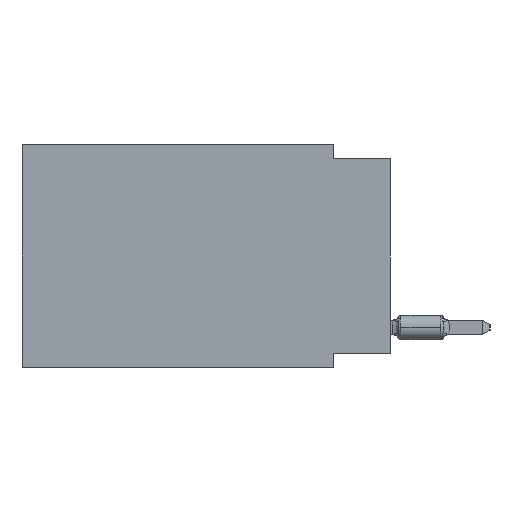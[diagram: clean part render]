
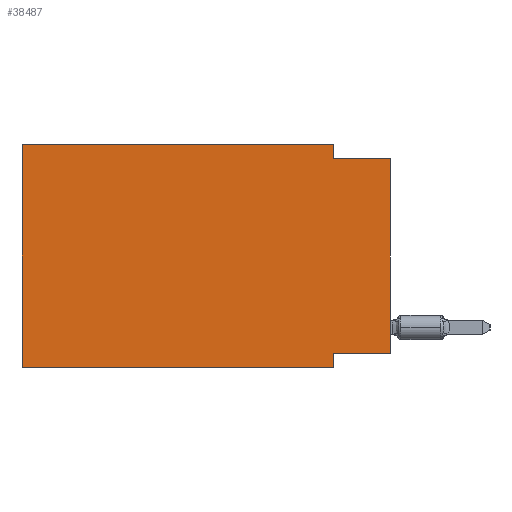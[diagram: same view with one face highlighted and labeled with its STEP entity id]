
A CAD part, left-side view. The second image highlights one B-rep face of the part: STEP entity #38487.
In plain terms, the highlighted planar face has unit normal (-1, 0, 0).
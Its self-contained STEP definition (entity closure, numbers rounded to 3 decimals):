
#952 = ORIENTED_EDGE ( 'NONE', *, *, #37551, .T. ) ;
#1107 = EDGE_CURVE ( 'NONE', #49571, #33872, #34606, .T. ) ;
#1662 = CARTESIAN_POINT ( 'NONE',  ( 0., 0., -0.635 ) ) ;
#1802 = CARTESIAN_POINT ( 'NONE',  ( 0., 16.383, -9.906 ) ) ;
#3372 = CARTESIAN_POINT ( 'NONE',  ( 0., 16.383, -9.906 ) ) ;
#3606 = CARTESIAN_POINT ( 'NONE',  ( 0., 16.383, 0. ) ) ;
#4074 = CARTESIAN_POINT ( 'NONE',  ( 0., 2.54, -9.906 ) ) ;
#4396 = CARTESIAN_POINT ( 'NONE',  ( 0., 16.383, 0. ) ) ;
#4826 = DIRECTION ( 'NONE',  ( 0., 0., -1. ) ) ;
#4965 = ORIENTED_EDGE ( 'NONE', *, *, #41860, .F. ) ;
#5560 = VECTOR ( 'NONE', #36702, 1000. ) ;
#5697 = VECTOR ( 'NONE', #9865, 1000. ) ;
#5885 = LINE ( 'NONE', #4396, #5697 ) ;
#6963 = VERTEX_POINT ( 'NONE', #3372 ) ;
#7174 = PLANE ( 'NONE',  #14794 ) ;
#7395 = ORIENTED_EDGE ( 'NONE', *, *, #29370, .F. ) ;
#7616 = ORIENTED_EDGE ( 'NONE', *, *, #27022, .F. ) ;
#8447 = CARTESIAN_POINT ( 'NONE',  ( 0., 2.54, -0.635 ) ) ;
#8450 = ORIENTED_EDGE ( 'NONE', *, *, #40389, .F. ) ;
#9865 = DIRECTION ( 'NONE',  ( 0., -1., 0. ) ) ;
#10168 = LINE ( 'NONE', #19240, #27542 ) ;
#10703 = DIRECTION ( 'NONE',  ( 0., 1., 0. ) ) ;
#12771 = LINE ( 'NONE', #24757, #39981 ) ;
#13487 = LINE ( 'NONE', #1802, #45988 ) ;
#13836 = LINE ( 'NONE', #37804, #19683 ) ;
#14794 = AXIS2_PLACEMENT_3D ( 'NONE', #23402, #39907, #47814 ) ;
#15162 = FACE_OUTER_BOUND ( 'NONE', #22699, .T. ) ;
#15617 = DIRECTION ( 'NONE',  ( 0., 0., 1. ) ) ;
#18920 = CARTESIAN_POINT ( 'NONE',  ( 0., 0., -0.635 ) ) ;
#19240 = CARTESIAN_POINT ( 'NONE',  ( 0., 0., -9.271 ) ) ;
#19683 = VECTOR ( 'NONE', #4826, 1000. ) ;
#19863 = CARTESIAN_POINT ( 'NONE',  ( 0., 16.383, 0. ) ) ;
#20728 = CARTESIAN_POINT ( 'NONE',  ( 0., 2.54, -9.906 ) ) ;
#21282 = ORIENTED_EDGE ( 'NONE', *, *, #37789, .F. ) ;
#21835 = CARTESIAN_POINT ( 'NONE',  ( 0., 2.54, -9.271 ) ) ;
#22699 = EDGE_LOOP ( 'NONE', ( #24700, #37128, #7616, #4965, #21282, #952, #7395, #8450 ) ) ;
#23038 = CARTESIAN_POINT ( 'NONE',  ( 0., 0., -9.271 ) ) ;
#23402 = CARTESIAN_POINT ( 'NONE',  ( 0., 16.383, 0. ) ) ;
#24357 = LINE ( 'NONE', #19863, #40078 ) ;
#24700 = ORIENTED_EDGE ( 'NONE', *, *, #46774, .T. ) ;
#24757 = CARTESIAN_POINT ( 'NONE',  ( 0., 0., 0. ) ) ;
#26623 = DIRECTION ( 'NONE',  ( 0., -1., 0. ) ) ;
#27022 = EDGE_CURVE ( 'NONE', #45020, #49571, #13836, .T. ) ;
#27542 = VECTOR ( 'NONE', #10703, 1000. ) ;
#28275 = CARTESIAN_POINT ( 'NONE',  ( 0., 2.54, 0. ) ) ;
#28503 = VERTEX_POINT ( 'NONE', #3606 ) ;
#29370 = EDGE_CURVE ( 'NONE', #40714, #30164, #45170, .T. ) ;
#30164 = VERTEX_POINT ( 'NONE', #4074 ) ;
#33008 = VECTOR ( 'NONE', #26623, 1000. ) ;
#33872 = VERTEX_POINT ( 'NONE', #1662 ) ;
#34606 = LINE ( 'NONE', #18920, #33008 ) ;
#36702 = DIRECTION ( 'NONE',  ( 0., 0., -1. ) ) ;
#37128 = ORIENTED_EDGE ( 'NONE', *, *, #1107, .F. ) ;
#37460 = DIRECTION ( 'NONE',  ( 0., -1., 0. ) ) ;
#37551 = EDGE_CURVE ( 'NONE', #6963, #30164, #13487, .T. ) ;
#37789 = EDGE_CURVE ( 'NONE', #6963, #28503, #24357, .T. ) ;
#37804 = CARTESIAN_POINT ( 'NONE',  ( 0., 2.54, 0. ) ) ;
#38487 = ADVANCED_FACE ( 'NONE', ( #15162 ), #7174, .F. ) ;
#39907 = DIRECTION ( 'NONE',  ( 1., 0., 0. ) ) ;
#39981 = VECTOR ( 'NONE', #40735, 1000. ) ;
#40078 = VECTOR ( 'NONE', #15617, 1000. ) ;
#40389 = EDGE_CURVE ( 'NONE', #42702, #40714, #10168, .T. ) ;
#40714 = VERTEX_POINT ( 'NONE', #21835 ) ;
#40735 = DIRECTION ( 'NONE',  ( 0., 0., 1. ) ) ;
#41860 = EDGE_CURVE ( 'NONE', #28503, #45020, #5885, .T. ) ;
#42702 = VERTEX_POINT ( 'NONE', #23038 ) ;
#45020 = VERTEX_POINT ( 'NONE', #28275 ) ;
#45170 = LINE ( 'NONE', #20728, #5560 ) ;
#45988 = VECTOR ( 'NONE', #37460, 1000. ) ;
#46774 = EDGE_CURVE ( 'NONE', #42702, #33872, #12771, .T. ) ;
#47814 = DIRECTION ( 'NONE',  ( 0., 0., -1. ) ) ;
#49571 = VERTEX_POINT ( 'NONE', #8447 ) ;
